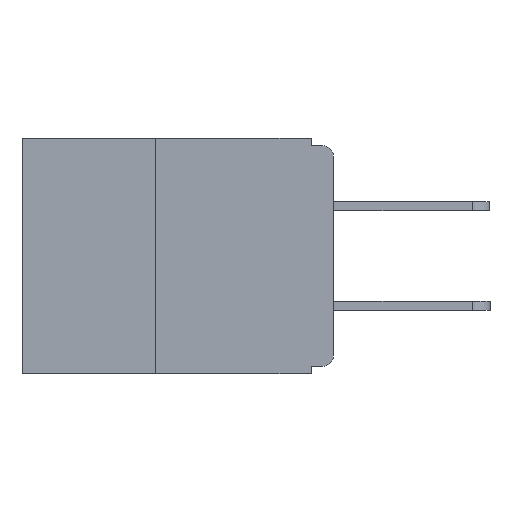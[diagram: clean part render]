
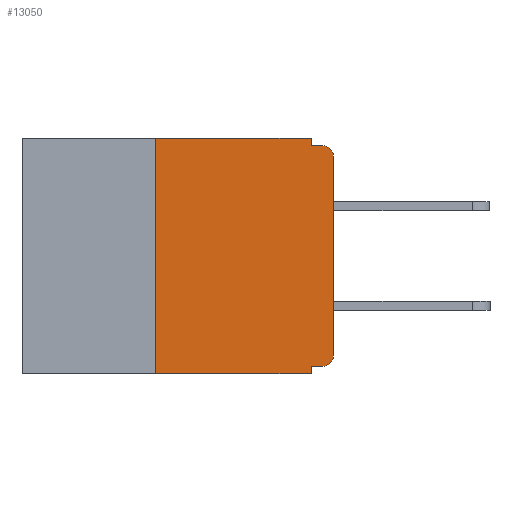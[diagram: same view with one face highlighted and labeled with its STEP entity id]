
A CAD part, left-side view. The second image highlights one B-rep face of the part: STEP entity #13050.
In plain terms, the highlighted planar face has unit normal (-1, 0, 0).
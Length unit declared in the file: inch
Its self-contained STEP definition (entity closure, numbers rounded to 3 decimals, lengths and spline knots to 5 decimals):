
#283 = VECTOR ( 'NONE', #1207, 39.37008 ) ;
#422 = DIRECTION ( 'NONE',  ( 0., 1., 0. ) ) ;
#447 = CARTESIAN_POINT ( 'NONE',  ( 0., 0., -0.32 ) ) ;
#524 = CARTESIAN_POINT ( 'NONE',  ( 0., 0., -0.025 ) ) ;
#540 = ORIENTED_EDGE ( 'NONE', *, *, #13702, .F. ) ;
#564 = DIRECTION ( 'NONE',  ( -1., 0., 0. ) ) ;
#1207 = DIRECTION ( 'NONE',  ( 0., 0., 1. ) ) ;
#1411 = CARTESIAN_POINT ( 'NONE',  ( 0., 0., 0. ) ) ;
#2052 = CARTESIAN_POINT ( 'NONE',  ( 0., 0.031, 0. ) ) ;
#2553 = CARTESIAN_POINT ( 'NONE',  ( 0., 0.437, -0.33 ) ) ;
#2597 = EDGE_LOOP ( 'NONE', ( #9933, #2972, #11176, #540, #15795, #9329, #12803, #9744, #16991, #14448 ) ) ;
#2745 = CARTESIAN_POINT ( 'NONE',  ( 0., 0.25, -0.33 ) ) ;
#2807 = AXIS2_PLACEMENT_3D ( 'NONE', #7010, #16171, #8397 ) ;
#2811 = CIRCLE ( 'NONE', #2807, 0.015 ) ;
#2972 = ORIENTED_EDGE ( 'NONE', *, *, #4205, .T. ) ;
#3185 = VERTEX_POINT ( 'NONE', #2745 ) ;
#3409 = CARTESIAN_POINT ( 'NONE',  ( 0., 0.437, 0. ) ) ;
#3447 = CARTESIAN_POINT ( 'NONE',  ( 0., 0.015, -0.01 ) ) ;
#4038 = VERTEX_POINT ( 'NONE', #11202 ) ;
#4087 = LINE ( 'NONE', #1411, #283 ) ;
#4205 = EDGE_CURVE ( 'NONE', #14264, #8669, #14615, .T. ) ;
#4322 = EDGE_CURVE ( 'NONE', #10491, #8635, #6432, .T. ) ;
#4719 = VECTOR ( 'NONE', #15504, 39.37008 ) ;
#4904 = CARTESIAN_POINT ( 'NONE',  ( 0., 0.031, 0. ) ) ;
#4979 = FACE_OUTER_BOUND ( 'NONE', #2597, .T. ) ;
#5573 = LINE ( 'NONE', #2553, #6014 ) ;
#6014 = VECTOR ( 'NONE', #12135, 39.37008 ) ;
#6315 = DIRECTION ( 'NONE',  ( 1., 0., 0. ) ) ;
#6358 = CARTESIAN_POINT ( 'NONE',  ( 0., 0.015, -0.025 ) ) ;
#6360 = LINE ( 'NONE', #9983, #9944 ) ;
#6432 = LINE ( 'NONE', #10847, #12669 ) ;
#6462 = VERTEX_POINT ( 'NONE', #9628 ) ;
#6699 = EDGE_CURVE ( 'NONE', #6462, #14264, #4087, .T. ) ;
#7010 = CARTESIAN_POINT ( 'NONE',  ( 0., 0.015, -0.305 ) ) ;
#7301 = LINE ( 'NONE', #8558, #16504 ) ;
#7948 = EDGE_CURVE ( 'NONE', #4038, #11531, #16546, .T. ) ;
#7998 = DIRECTION ( 'NONE',  ( 0., 0., -1. ) ) ;
#8397 = DIRECTION ( 'NONE',  ( 0., 0., -1. ) ) ;
#8402 = LINE ( 'NONE', #2052, #4719 ) ;
#8558 = CARTESIAN_POINT ( 'NONE',  ( 0., 0.031, -0.33 ) ) ;
#8635 = VERTEX_POINT ( 'NONE', #4904 ) ;
#8669 = VERTEX_POINT ( 'NONE', #3447 ) ;
#8706 = CARTESIAN_POINT ( 'NONE',  ( 0., 0.031, -0.01 ) ) ;
#8984 = AXIS2_PLACEMENT_3D ( 'NONE', #3409, #6315, #15522 ) ;
#9085 = DIRECTION ( 'NONE',  ( 0., -1., 0. ) ) ;
#9314 = EDGE_CURVE ( 'NONE', #11531, #10501, #7301, .T. ) ;
#9329 = ORIENTED_EDGE ( 'NONE', *, *, #11077, .F. ) ;
#9609 = DIRECTION ( 'NONE',  ( 0., -1., 0. ) ) ;
#9628 = CARTESIAN_POINT ( 'NONE',  ( 0., 0., -0.305 ) ) ;
#9706 = VECTOR ( 'NONE', #422, 39.37008 ) ;
#9744 = ORIENTED_EDGE ( 'NONE', *, *, #9314, .F. ) ;
#9933 = ORIENTED_EDGE ( 'NONE', *, *, #6699, .T. ) ;
#9944 = VECTOR ( 'NONE', #11312, 39.37008 ) ;
#9983 = CARTESIAN_POINT ( 'NONE',  ( 0., 0.25, -0.33 ) ) ;
#10199 = EDGE_CURVE ( 'NONE', #3185, #10501, #5573, .T. ) ;
#10491 = VERTEX_POINT ( 'NONE', #14000 ) ;
#10501 = VERTEX_POINT ( 'NONE', #12742 ) ;
#10847 = CARTESIAN_POINT ( 'NONE',  ( 0., 0.437, 0. ) ) ;
#11077 = EDGE_CURVE ( 'NONE', #3185, #10491, #6360, .T. ) ;
#11176 = ORIENTED_EDGE ( 'NONE', *, *, #15825, .F. ) ;
#11202 = CARTESIAN_POINT ( 'NONE',  ( 0., 0.015, -0.32 ) ) ;
#11312 = DIRECTION ( 'NONE',  ( 0., 0., 1. ) ) ;
#11531 = VERTEX_POINT ( 'NONE', #14826 ) ;
#12135 = DIRECTION ( 'NONE',  ( 0., -1., 0. ) ) ;
#12190 = CARTESIAN_POINT ( 'NONE',  ( 0., 0., -0.01 ) ) ;
#12438 = VECTOR ( 'NONE', #9609, 39.37008 ) ;
#12669 = VECTOR ( 'NONE', #9085, 39.37008 ) ;
#12742 = CARTESIAN_POINT ( 'NONE',  ( 0., 0.031, -0.33 ) ) ;
#12803 = ORIENTED_EDGE ( 'NONE', *, *, #10199, .T. ) ;
#12850 = LINE ( 'NONE', #12190, #12438 ) ;
#12902 = VERTEX_POINT ( 'NONE', #8706 ) ;
#13050 = ADVANCED_FACE ( 'NONE', ( #4979 ), #16725, .F. ) ;
#13702 = EDGE_CURVE ( 'NONE', #8635, #12902, #8402, .T. ) ;
#14000 = CARTESIAN_POINT ( 'NONE',  ( 0., 0.25, 0. ) ) ;
#14121 = AXIS2_PLACEMENT_3D ( 'NONE', #6358, #564, #16173 ) ;
#14264 = VERTEX_POINT ( 'NONE', #524 ) ;
#14448 = ORIENTED_EDGE ( 'NONE', *, *, #16996, .T. ) ;
#14615 = CIRCLE ( 'NONE', #14121, 0.015 ) ;
#14826 = CARTESIAN_POINT ( 'NONE',  ( 0., 0.031, -0.32 ) ) ;
#15504 = DIRECTION ( 'NONE',  ( 0., 0., -1. ) ) ;
#15522 = DIRECTION ( 'NONE',  ( 0., 0., -1. ) ) ;
#15795 = ORIENTED_EDGE ( 'NONE', *, *, #4322, .F. ) ;
#15825 = EDGE_CURVE ( 'NONE', #12902, #8669, #12850, .T. ) ;
#16171 = DIRECTION ( 'NONE',  ( -1., 0., 0. ) ) ;
#16173 = DIRECTION ( 'NONE',  ( 0., 0., -1. ) ) ;
#16504 = VECTOR ( 'NONE', #7998, 39.37008 ) ;
#16546 = LINE ( 'NONE', #447, #9706 ) ;
#16725 = PLANE ( 'NONE',  #8984 ) ;
#16991 = ORIENTED_EDGE ( 'NONE', *, *, #7948, .F. ) ;
#16996 = EDGE_CURVE ( 'NONE', #4038, #6462, #2811, .T. ) ;
